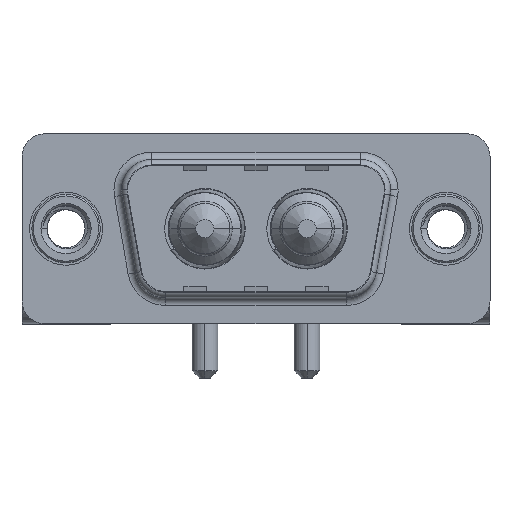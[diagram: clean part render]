
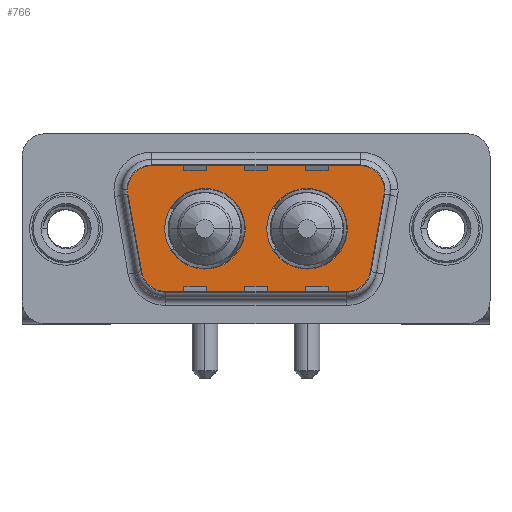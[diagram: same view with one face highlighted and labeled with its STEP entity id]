
A CAD part, top view. The second image highlights one B-rep face of the part: STEP entity #766.
In plain terms, the highlighted planar face has unit normal (0, 0, 1).
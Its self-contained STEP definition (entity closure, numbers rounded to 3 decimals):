
#108 = VERTEX_POINT ( 'NONE', #4607 ) ;
#315 = VERTEX_POINT ( 'NONE', #10820 ) ;
#374 = CIRCLE ( 'NONE', #3792, 2. ) ;
#621 = CARTESIAN_POINT ( 'NONE',  ( 9.14, 0., 0. ) ) ;
#732 = EDGE_CURVE ( 'NONE', #1046, #2743, #12688, .T. ) ;
#766 = ADVANCED_FACE ( 'NONE', ( #1624, #10309, #10245 ), #2552, .T. ) ;
#795 = CARTESIAN_POINT ( 'NONE',  ( 21.564, 2.9, 0. ) ) ;
#947 = CARTESIAN_POINT ( 'NONE',  ( 18.541, -4.9, 0. ) ) ;
#1046 = VERTEX_POINT ( 'NONE', #2059 ) ;
#1500 = VECTOR ( 'NONE', #9901, 1000. ) ;
#1624 = FACE_BOUND ( 'NONE', #3854, .T. ) ;
#1648 = CARTESIAN_POINT ( 'NONE',  ( 19.564, 2.9, 0. ) ) ;
#1869 = CIRCLE ( 'NONE', #9840, 2. ) ;
#1910 = EDGE_CURVE ( 'NONE', #9952, #9567, #2393, .T. ) ;
#2059 = CARTESIAN_POINT ( 'NONE',  ( 11.79, 0., 0. ) ) ;
#2072 = CARTESIAN_POINT ( 'NONE',  ( 21.534, 2.553, 0. ) ) ;
#2271 = VECTOR ( 'NONE', #3259, 1000. ) ;
#2363 = CARTESIAN_POINT ( 'NONE',  ( 5.436, 4.9, 0. ) ) ;
#2393 = CIRCLE ( 'NONE', #4213, 2. ) ;
#2458 = VECTOR ( 'NONE', #10460, 1000. ) ;
#2552 = PLANE ( 'NONE',  #4976 ) ;
#2629 = ORIENTED_EDGE ( 'NONE', *, *, #732, .F. ) ;
#2707 = AXIS2_PLACEMENT_3D ( 'NONE', #621, #5827, #6967 ) ;
#2743 = VERTEX_POINT ( 'NONE', #11701 ) ;
#2768 = EDGE_LOOP ( 'NONE', ( #2629, #5071 ) ) ;
#2817 = DIRECTION ( 'NONE',  ( 0., 0., 1. ) ) ;
#3091 = EDGE_CURVE ( 'NONE', #13876, #4832, #3521, .T. ) ;
#3136 = CIRCLE ( 'NONE', #4291, 2.65 ) ;
#3171 = CIRCLE ( 'NONE', #11130, 2. ) ;
#3233 = ORIENTED_EDGE ( 'NONE', *, *, #1910, .T. ) ;
#3259 = DIRECTION ( 'NONE',  ( 0.174, -0.985, 0. ) ) ;
#3331 = DIRECTION ( 'NONE',  ( 1., 0., 0. ) ) ;
#3521 = LINE ( 'NONE', #11133, #6047 ) ;
#3792 = AXIS2_PLACEMENT_3D ( 'NONE', #11795, #4266, #8598 ) ;
#3814 = DIRECTION ( 'NONE',  ( 1., 0., 0. ) ) ;
#3820 = EDGE_CURVE ( 'NONE', #9567, #108, #374, .T. ) ;
#3854 = EDGE_LOOP ( 'NONE', ( #13269, #11092 ) ) ;
#4171 = CIRCLE ( 'NONE', #12114, 2. ) ;
#4186 = ORIENTED_EDGE ( 'NONE', *, *, #13039, .T. ) ;
#4213 = AXIS2_PLACEMENT_3D ( 'NONE', #1648, #7331, #12790 ) ;
#4266 = DIRECTION ( 'NONE',  ( 0., 0., 1. ) ) ;
#4291 = AXIS2_PLACEMENT_3D ( 'NONE', #7245, #10524, #3331 ) ;
#4383 = ORIENTED_EDGE ( 'NONE', *, *, #8588, .T. ) ;
#4525 = DIRECTION ( 'NONE',  ( 0., 0., 1. ) ) ;
#4607 = CARTESIAN_POINT ( 'NONE',  ( 19.564, 4.9, 0. ) ) ;
#4609 = CIRCLE ( 'NONE', #8709, 2.65 ) ;
#4638 = ORIENTED_EDGE ( 'NONE', *, *, #10151, .T. ) ;
#4832 = VERTEX_POINT ( 'NONE', #947 ) ;
#4976 = AXIS2_PLACEMENT_3D ( 'NONE', #4977, #10169, #11172 ) ;
#4977 = CARTESIAN_POINT ( 'NONE',  ( 18.541, -2.9, 0. ) ) ;
#5071 = ORIENTED_EDGE ( 'NONE', *, *, #10358, .F. ) ;
#5298 = CIRCLE ( 'NONE', #13929, 2.65 ) ;
#5598 = CARTESIAN_POINT ( 'NONE',  ( 20.511, -3.247, 0. ) ) ;
#5827 = DIRECTION ( 'NONE',  ( 0., 0., 1. ) ) ;
#5829 = DIRECTION ( 'NONE',  ( 0., 0., 1. ) ) ;
#6047 = VECTOR ( 'NONE', #6993, 1000. ) ;
#6051 = VERTEX_POINT ( 'NONE', #10578 ) ;
#6073 = CARTESIAN_POINT ( 'NONE',  ( 5.436, 4.9, 0. ) ) ;
#6266 = DIRECTION ( 'NONE',  ( 1., 0., 0. ) ) ;
#6337 = DIRECTION ( 'NONE',  ( 0., 0., 1. ) ) ;
#6427 = EDGE_CURVE ( 'NONE', #108, #10629, #8833, .T. ) ;
#6655 = EDGE_LOOP ( 'NONE', ( #4638, #4186, #3233, #8923, #12890, #8820, #4383, #7114, #8215 ) ) ;
#6841 = DIRECTION ( 'NONE',  ( 0., 0., 1. ) ) ;
#6967 = DIRECTION ( 'NONE',  ( 1., 0., 0. ) ) ;
#6993 = DIRECTION ( 'NONE',  ( 1., 0., 0. ) ) ;
#7114 = ORIENTED_EDGE ( 'NONE', *, *, #8972, .T. ) ;
#7245 = CARTESIAN_POINT ( 'NONE',  ( 15.86, 0., 0. ) ) ;
#7331 = DIRECTION ( 'NONE',  ( 0., 0., 1. ) ) ;
#7588 = DIRECTION ( 'NONE',  ( 1., 0., 0. ) ) ;
#8096 = VERTEX_POINT ( 'NONE', #11946 ) ;
#8215 = ORIENTED_EDGE ( 'NONE', *, *, #3091, .T. ) ;
#8588 = EDGE_CURVE ( 'NONE', #315, #8096, #12917, .T. ) ;
#8598 = DIRECTION ( 'NONE',  ( -1., 0., 0. ) ) ;
#8709 = AXIS2_PLACEMENT_3D ( 'NONE', #9927, #4525, #7588 ) ;
#8820 = ORIENTED_EDGE ( 'NONE', *, *, #11645, .T. ) ;
#8833 = LINE ( 'NONE', #2363, #1500 ) ;
#8923 = ORIENTED_EDGE ( 'NONE', *, *, #3820, .T. ) ;
#8972 = EDGE_CURVE ( 'NONE', #8096, #13876, #3171, .T. ) ;
#9035 = CARTESIAN_POINT ( 'NONE',  ( 18.541, -2.9, 0. ) ) ;
#9296 = DIRECTION ( 'NONE',  ( -1., 0., 0. ) ) ;
#9378 = VERTEX_POINT ( 'NONE', #10271 ) ;
#9567 = VERTEX_POINT ( 'NONE', #795 ) ;
#9840 = AXIS2_PLACEMENT_3D ( 'NONE', #9035, #6841, #3814 ) ;
#9901 = DIRECTION ( 'NONE',  ( -1., 0., 0. ) ) ;
#9927 = CARTESIAN_POINT ( 'NONE',  ( 9.14, 0., 0. ) ) ;
#9952 = VERTEX_POINT ( 'NONE', #2072 ) ;
#10151 = EDGE_CURVE ( 'NONE', #4832, #13986, #1869, .T. ) ;
#10169 = DIRECTION ( 'NONE',  ( 0., 0., 1. ) ) ;
#10245 = FACE_OUTER_BOUND ( 'NONE', #6655, .T. ) ;
#10271 = CARTESIAN_POINT ( 'NONE',  ( 13.21, 0., 0. ) ) ;
#10309 = FACE_BOUND ( 'NONE', #2768, .T. ) ;
#10310 = DIRECTION ( 'NONE',  ( 1., 0., 0. ) ) ;
#10358 = EDGE_CURVE ( 'NONE', #2743, #1046, #4609, .T. ) ;
#10460 = DIRECTION ( 'NONE',  ( 0.174, 0.985, 0. ) ) ;
#10524 = DIRECTION ( 'NONE',  ( 0., 0., 1. ) ) ;
#10578 = CARTESIAN_POINT ( 'NONE',  ( 18.51, 0., 0. ) ) ;
#10629 = VERTEX_POINT ( 'NONE', #6073 ) ;
#10820 = CARTESIAN_POINT ( 'NONE',  ( 3.466, 2.553, 0. ) ) ;
#11092 = ORIENTED_EDGE ( 'NONE', *, *, #13174, .F. ) ;
#11126 = EDGE_CURVE ( 'NONE', #6051, #9378, #5298, .T. ) ;
#11130 = AXIS2_PLACEMENT_3D ( 'NONE', #12613, #2817, #9296 ) ;
#11133 = CARTESIAN_POINT ( 'NONE',  ( 6.459, -4.9, 0. ) ) ;
#11172 = DIRECTION ( 'NONE',  ( 1., 0., 0. ) ) ;
#11237 = CARTESIAN_POINT ( 'NONE',  ( 15.86, 0., 0. ) ) ;
#11645 = EDGE_CURVE ( 'NONE', #10629, #315, #4171, .T. ) ;
#11658 = LINE ( 'NONE', #13655, #2458 ) ;
#11676 = CARTESIAN_POINT ( 'NONE',  ( 5.436, 2.9, 0. ) ) ;
#11701 = CARTESIAN_POINT ( 'NONE',  ( 6.49, 0., 0. ) ) ;
#11795 = CARTESIAN_POINT ( 'NONE',  ( 19.564, 2.9, 0. ) ) ;
#11946 = CARTESIAN_POINT ( 'NONE',  ( 4.489, -3.247, 0. ) ) ;
#12114 = AXIS2_PLACEMENT_3D ( 'NONE', #11676, #6337, #6266 ) ;
#12613 = CARTESIAN_POINT ( 'NONE',  ( 6.459, -2.9, 0. ) ) ;
#12688 = CIRCLE ( 'NONE', #2707, 2.65 ) ;
#12790 = DIRECTION ( 'NONE',  ( -1., 0., 0. ) ) ;
#12890 = ORIENTED_EDGE ( 'NONE', *, *, #6427, .T. ) ;
#12917 = LINE ( 'NONE', #12991, #2271 ) ;
#12991 = CARTESIAN_POINT ( 'NONE',  ( 3.466, 2.553, 0. ) ) ;
#13039 = EDGE_CURVE ( 'NONE', #13986, #9952, #11658, .T. ) ;
#13174 = EDGE_CURVE ( 'NONE', #9378, #6051, #3136, .T. ) ;
#13269 = ORIENTED_EDGE ( 'NONE', *, *, #11126, .F. ) ;
#13427 = CARTESIAN_POINT ( 'NONE',  ( 6.459, -4.9, 0. ) ) ;
#13655 = CARTESIAN_POINT ( 'NONE',  ( 21.534, 2.553, 0. ) ) ;
#13876 = VERTEX_POINT ( 'NONE', #13427 ) ;
#13929 = AXIS2_PLACEMENT_3D ( 'NONE', #11237, #5829, #10310 ) ;
#13986 = VERTEX_POINT ( 'NONE', #5598 ) ;
